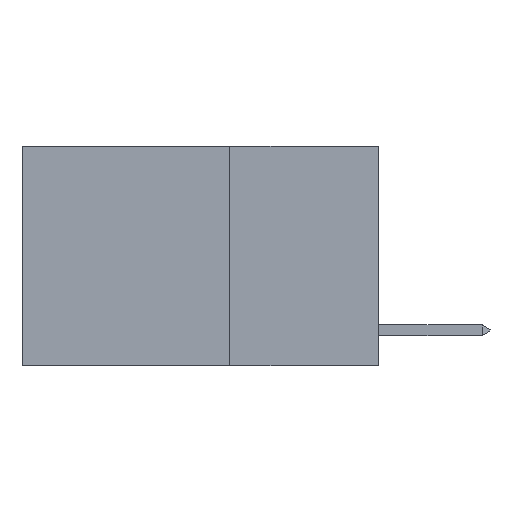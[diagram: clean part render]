
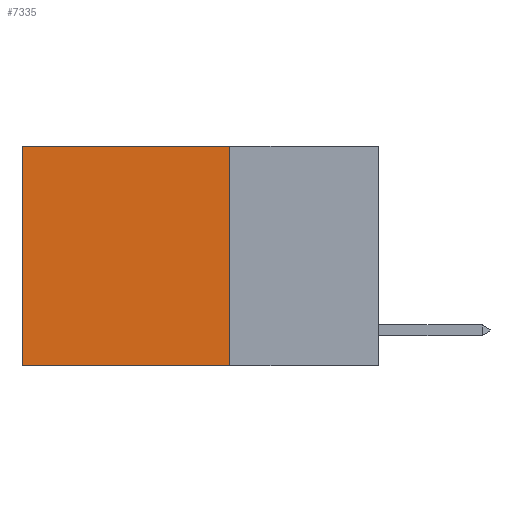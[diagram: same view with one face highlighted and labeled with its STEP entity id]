
A CAD part, left-side view. The second image highlights one B-rep face of the part: STEP entity #7335.
In plain terms, the highlighted planar face has unit normal (-1, 0, 0).
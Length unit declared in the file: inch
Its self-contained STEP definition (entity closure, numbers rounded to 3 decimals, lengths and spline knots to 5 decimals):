
#1236 = CARTESIAN_POINT ( 'NONE',  ( 0.2625, 0.6, -0.37 ) ) ;
#1713 = VERTEX_POINT ( 'NONE', #7916 ) ;
#1798 = VECTOR ( 'NONE', #5302, 39.37008 ) ;
#2045 = ORIENTED_EDGE ( 'NONE', *, *, #4810, .F. ) ;
#3304 = DIRECTION ( 'NONE',  ( 1., 0., 0. ) ) ;
#4810 = EDGE_CURVE ( 'NONE', #5171, #1713, #13330, .T. ) ;
#4858 = CARTESIAN_POINT ( 'NONE',  ( 0.2625, 0.6, 0. ) ) ;
#4891 = VERTEX_POINT ( 'NONE', #1236 ) ;
#5171 = VERTEX_POINT ( 'NONE', #8241 ) ;
#5302 = DIRECTION ( 'NONE',  ( 0., 0., -1. ) ) ;
#5561 = VECTOR ( 'NONE', #11492, 39.37008 ) ;
#5871 = FACE_OUTER_BOUND ( 'NONE', #7331, .T. ) ;
#5890 = CARTESIAN_POINT ( 'NONE',  ( 0.2625, 0.25, 0. ) ) ;
#6286 = ORIENTED_EDGE ( 'NONE', *, *, #11737, .T. ) ;
#7331 = EDGE_LOOP ( 'NONE', ( #6286, #9451, #2045, #16354 ) ) ;
#7335 = ADVANCED_FACE ( 'NONE', ( #5871 ), #17614, .F. ) ;
#7825 = LINE ( 'NONE', #13837, #1798 ) ;
#7916 = CARTESIAN_POINT ( 'NONE',  ( 0.2625, 0.25, -0.37 ) ) ;
#8241 = CARTESIAN_POINT ( 'NONE',  ( 0.2625, 0.25, 0. ) ) ;
#8664 = LINE ( 'NONE', #5890, #5561 ) ;
#9451 = ORIENTED_EDGE ( 'NONE', *, *, #15323, .F. ) ;
#10508 = AXIS2_PLACEMENT_3D ( 'NONE', #11850, #3304, #13161 ) ;
#11492 = DIRECTION ( 'NONE',  ( 0., 1., 0. ) ) ;
#11737 = EDGE_CURVE ( 'NONE', #17019, #4891, #7825, .T. ) ;
#11850 = CARTESIAN_POINT ( 'NONE',  ( 0.2625, 0.25, 0. ) ) ;
#13161 = DIRECTION ( 'NONE',  ( 0., 0., -1. ) ) ;
#13330 = LINE ( 'NONE', #14581, #18207 ) ;
#13837 = CARTESIAN_POINT ( 'NONE',  ( 0.2625, 0.6, 0. ) ) ;
#14581 = CARTESIAN_POINT ( 'NONE',  ( 0.2625, 0.25, 0. ) ) ;
#15323 = EDGE_CURVE ( 'NONE', #1713, #4891, #15461, .T. ) ;
#15358 = CARTESIAN_POINT ( 'NONE',  ( 0.2625, 0.25, -0.37 ) ) ;
#15461 = LINE ( 'NONE', #15358, #15676 ) ;
#15676 = VECTOR ( 'NONE', #18019, 39.37008 ) ;
#15867 = DIRECTION ( 'NONE',  ( 0., 0., -1. ) ) ;
#16354 = ORIENTED_EDGE ( 'NONE', *, *, #18381, .T. ) ;
#17019 = VERTEX_POINT ( 'NONE', #4858 ) ;
#17614 = PLANE ( 'NONE',  #10508 ) ;
#18019 = DIRECTION ( 'NONE',  ( 0., 1., 0. ) ) ;
#18207 = VECTOR ( 'NONE', #15867, 39.37008 ) ;
#18381 = EDGE_CURVE ( 'NONE', #5171, #17019, #8664, .T. ) ;
